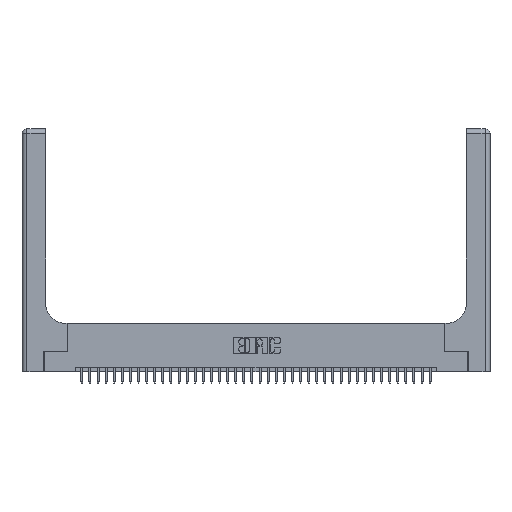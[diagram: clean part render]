
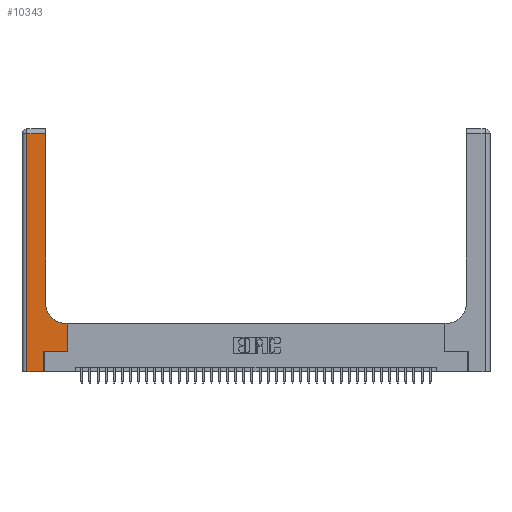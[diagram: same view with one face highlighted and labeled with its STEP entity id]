
A CAD part, top view. The second image highlights one B-rep face of the part: STEP entity #10343.
In plain terms, the highlighted planar face has unit normal (0, 0, 1).
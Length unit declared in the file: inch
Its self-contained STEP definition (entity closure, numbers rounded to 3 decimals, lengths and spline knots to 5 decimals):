
#833 = VERTEX_POINT ( 'NONE', #18007 ) ;
#1059 = ORIENTED_EDGE ( 'NONE', *, *, #7110, .T. ) ;
#1549 = CARTESIAN_POINT ( 'NONE',  ( 0.269, 0., 0.37 ) ) ;
#1674 = VECTOR ( 'NONE', #13641, 39.37008 ) ;
#1975 = CARTESIAN_POINT ( 'NONE',  ( 0.269, 0.25, 0.37 ) ) ;
#3010 = VECTOR ( 'NONE', #12179, 39.37008 ) ;
#3971 = EDGE_CURVE ( 'NONE', #30496, #26073, #18987, .T. ) ;
#4000 = CARTESIAN_POINT ( 'NONE',  ( 0.06, 2.94, 0.37 ) ) ;
#4327 = ORIENTED_EDGE ( 'NONE', *, *, #27091, .T. ) ;
#5668 = VERTEX_POINT ( 'NONE', #24946 ) ;
#5889 = VECTOR ( 'NONE', #33450, 39.37008 ) ;
#5985 = ORIENTED_EDGE ( 'NONE', *, *, #18845, .T. ) ;
#6276 = EDGE_LOOP ( 'NONE', ( #1059, #4327, #37952, #31065, #24224, #23101, #12276, #5985, #13298 ) ) ;
#7110 = EDGE_CURVE ( 'NONE', #12970, #5668, #33116, .T. ) ;
#7796 = AXIS2_PLACEMENT_3D ( 'NONE', #8468, #29784, #11531 ) ;
#8293 = DIRECTION ( 'NONE',  ( 1., 0., 0. ) ) ;
#8468 = CARTESIAN_POINT ( 'NONE',  ( 0.5415, 0.85, 0.37 ) ) ;
#9143 = CARTESIAN_POINT ( 'NONE',  ( 0.5585, 0.25, 0.37 ) ) ;
#9929 = LINE ( 'NONE', #15144, #25149 ) ;
#10343 = ADVANCED_FACE ( 'NONE', ( #37472 ), #14431, .F. ) ;
#11531 = DIRECTION ( 'NONE',  ( 1., 0., 0. ) ) ;
#11539 = LINE ( 'NONE', #12912, #34877 ) ;
#12037 = DIRECTION ( 'NONE',  ( -1., 0., 0. ) ) ;
#12179 = DIRECTION ( 'NONE',  ( 0., 1., 0. ) ) ;
#12276 = ORIENTED_EDGE ( 'NONE', *, *, #20694, .T. ) ;
#12826 = EDGE_CURVE ( 'NONE', #32495, #833, #15311, .T. ) ;
#12912 = CARTESIAN_POINT ( 'NONE',  ( 0., 2.94, 0.37 ) ) ;
#12970 = VERTEX_POINT ( 'NONE', #18819 ) ;
#13298 = ORIENTED_EDGE ( 'NONE', *, *, #16976, .T. ) ;
#13641 = DIRECTION ( 'NONE',  ( 0., 1., 0. ) ) ;
#14431 = PLANE ( 'NONE',  #32625 ) ;
#15144 = CARTESIAN_POINT ( 'NONE',  ( 0., 0., 0.37 ) ) ;
#15166 = CARTESIAN_POINT ( 'NONE',  ( 0.269, 0.25, 0.37 ) ) ;
#15311 = LINE ( 'NONE', #18174, #31564 ) ;
#16976 = EDGE_CURVE ( 'NONE', #38814, #12970, #34762, .T. ) ;
#17513 = DIRECTION ( 'NONE',  ( 0., 0., -1. ) ) ;
#17740 = EDGE_CURVE ( 'NONE', #833, #30496, #9929, .T. ) ;
#18007 = CARTESIAN_POINT ( 'NONE',  ( 0.06, 0., 0.37 ) ) ;
#18174 = CARTESIAN_POINT ( 'NONE',  ( 0.06, 3., 0.37 ) ) ;
#18819 = CARTESIAN_POINT ( 'NONE',  ( 0.2915, 0.85, 0.37 ) ) ;
#18845 = EDGE_CURVE ( 'NONE', #34417, #38814, #29407, .T. ) ;
#18987 = LINE ( 'NONE', #1549, #37114 ) ;
#19032 = CARTESIAN_POINT ( 'NONE',  ( 0.5415, 0.6, 0.37 ) ) ;
#20694 = EDGE_CURVE ( 'NONE', #37040, #34417, #27322, .T. ) ;
#21360 = EDGE_CURVE ( 'NONE', #26073, #37040, #37734, .T. ) ;
#22876 = DIRECTION ( 'NONE',  ( 0., 1., 0. ) ) ;
#23101 = ORIENTED_EDGE ( 'NONE', *, *, #21360, .T. ) ;
#24224 = ORIENTED_EDGE ( 'NONE', *, *, #3971, .T. ) ;
#24946 = CARTESIAN_POINT ( 'NONE',  ( 0.2915, 2.94, 0.37 ) ) ;
#25149 = VECTOR ( 'NONE', #8293, 39.37008 ) ;
#26073 = VERTEX_POINT ( 'NONE', #1975 ) ;
#27091 = EDGE_CURVE ( 'NONE', #5668, #32495, #11539, .T. ) ;
#27222 = CARTESIAN_POINT ( 'NONE',  ( 0.2915, 0.6, 0.37 ) ) ;
#27272 = DIRECTION ( 'NONE',  ( 0., -1., 0. ) ) ;
#27322 = LINE ( 'NONE', #9143, #3010 ) ;
#28879 = CARTESIAN_POINT ( 'NONE',  ( 0.2915, 3., 0.37 ) ) ;
#29407 = LINE ( 'NONE', #27222, #36501 ) ;
#29531 = CARTESIAN_POINT ( 'NONE',  ( 0.269, 0., 0.37 ) ) ;
#29784 = DIRECTION ( 'NONE',  ( 0., 0., -1. ) ) ;
#30496 = VERTEX_POINT ( 'NONE', #29531 ) ;
#31065 = ORIENTED_EDGE ( 'NONE', *, *, #17740, .T. ) ;
#31199 = DIRECTION ( 'NONE',  ( -1., 0., 0. ) ) ;
#31319 = CARTESIAN_POINT ( 'NONE',  ( 0.5585, 0.6, 0.37 ) ) ;
#31564 = VECTOR ( 'NONE', #27272, 39.37008 ) ;
#32495 = VERTEX_POINT ( 'NONE', #4000 ) ;
#32625 = AXIS2_PLACEMENT_3D ( 'NONE', #35776, #17513, #38845 ) ;
#33116 = LINE ( 'NONE', #28879, #1674 ) ;
#33450 = DIRECTION ( 'NONE',  ( 1., 0., 0. ) ) ;
#34417 = VERTEX_POINT ( 'NONE', #31319 ) ;
#34762 = CIRCLE ( 'NONE', #7796, 0.25 ) ;
#34877 = VECTOR ( 'NONE', #31199, 39.37008 ) ;
#35776 = CARTESIAN_POINT ( 'NONE',  ( 0., 3., 0.37 ) ) ;
#36501 = VECTOR ( 'NONE', #12037, 39.37008 ) ;
#37040 = VERTEX_POINT ( 'NONE', #37455 ) ;
#37114 = VECTOR ( 'NONE', #22876, 39.37008 ) ;
#37455 = CARTESIAN_POINT ( 'NONE',  ( 0.5585, 0.25, 0.37 ) ) ;
#37472 = FACE_OUTER_BOUND ( 'NONE', #6276, .T. ) ;
#37734 = LINE ( 'NONE', #15166, #5889 ) ;
#37952 = ORIENTED_EDGE ( 'NONE', *, *, #12826, .T. ) ;
#38814 = VERTEX_POINT ( 'NONE', #19032 ) ;
#38845 = DIRECTION ( 'NONE',  ( -1., 0., 0. ) ) ;
